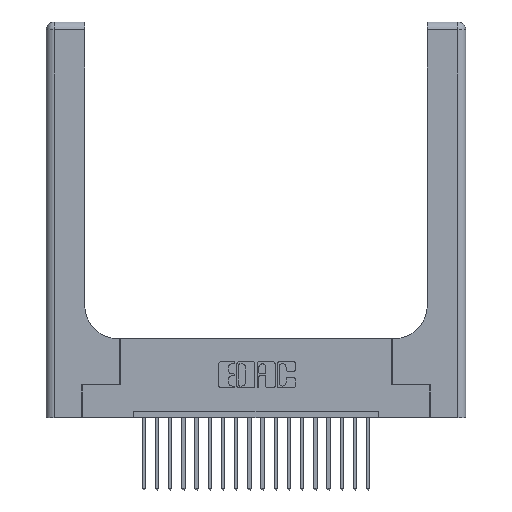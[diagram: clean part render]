
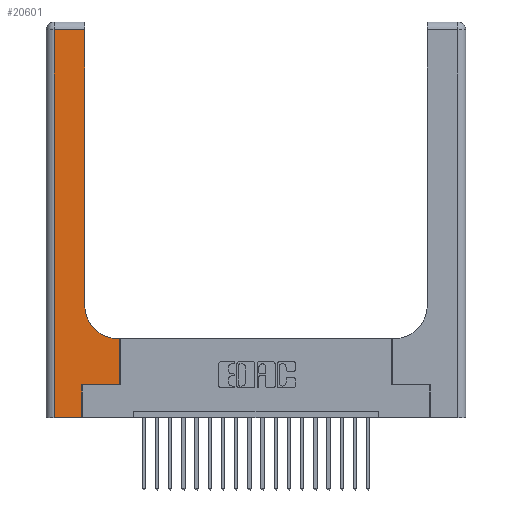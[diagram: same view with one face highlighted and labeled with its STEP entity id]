
A CAD part, top view. The second image highlights one B-rep face of the part: STEP entity #20601.
In plain terms, the highlighted planar face has unit normal (0, 0, 1).
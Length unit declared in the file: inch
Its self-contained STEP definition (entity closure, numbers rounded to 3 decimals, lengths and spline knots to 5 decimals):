
#178 = LINE ( 'NONE', #3616, #10023 ) ;
#368 = EDGE_CURVE ( 'NONE', #13290, #6331, #4164, .T. ) ;
#420 = CARTESIAN_POINT ( 'NONE',  ( 0.06, 3., 0.37 ) ) ;
#850 = AXIS2_PLACEMENT_3D ( 'NONE', #21182, #11050, #14389 ) ;
#1238 = VECTOR ( 'NONE', #5958, 39.37008 ) ;
#1282 = EDGE_CURVE ( 'NONE', #18139, #15798, #9683, .T. ) ;
#2224 = ORIENTED_EDGE ( 'NONE', *, *, #4259, .T. ) ;
#2314 = VECTOR ( 'NONE', #4105, 39.37008 ) ;
#2842 = VERTEX_POINT ( 'NONE', #9582 ) ;
#3616 = CARTESIAN_POINT ( 'NONE',  ( 0.269, 0., 0.37 ) ) ;
#3642 = CARTESIAN_POINT ( 'NONE',  ( 0.06, 0., 0.37 ) ) ;
#3695 = CARTESIAN_POINT ( 'NONE',  ( 0.2915, 3., 0.37 ) ) ;
#3756 = EDGE_LOOP ( 'NONE', ( #5362, #13397, #7333, #3832, #2224, #4231, #17877, #12104, #7374 ) ) ;
#3794 = VECTOR ( 'NONE', #12310, 39.37008 ) ;
#3820 = DIRECTION ( 'NONE',  ( -1., 0., 0. ) ) ;
#3832 = ORIENTED_EDGE ( 'NONE', *, *, #6887, .T. ) ;
#4105 = DIRECTION ( 'NONE',  ( 0., 1., 0. ) ) ;
#4164 = LINE ( 'NONE', #3695, #2314 ) ;
#4189 = EDGE_CURVE ( 'NONE', #15798, #5351, #21672, .T. ) ;
#4231 = ORIENTED_EDGE ( 'NONE', *, *, #1282, .T. ) ;
#4244 = VERTEX_POINT ( 'NONE', #17295 ) ;
#4259 = EDGE_CURVE ( 'NONE', #2842, #18139, #178, .T. ) ;
#4546 = CARTESIAN_POINT ( 'NONE',  ( 0.5585, 0.25, 0.37 ) ) ;
#5351 = VERTEX_POINT ( 'NONE', #12432 ) ;
#5362 = ORIENTED_EDGE ( 'NONE', *, *, #368, .T. ) ;
#5958 = DIRECTION ( 'NONE',  ( 1., 0., 0. ) ) ;
#6331 = VERTEX_POINT ( 'NONE', #7026 ) ;
#6453 = CARTESIAN_POINT ( 'NONE',  ( 0.2915, 0.85, 0.37 ) ) ;
#6887 = EDGE_CURVE ( 'NONE', #18558, #2842, #7539, .T. ) ;
#7026 = CARTESIAN_POINT ( 'NONE',  ( 0.2915, 2.94, 0.37 ) ) ;
#7333 = ORIENTED_EDGE ( 'NONE', *, *, #8013, .T. ) ;
#7374 = ORIENTED_EDGE ( 'NONE', *, *, #14523, .T. ) ;
#7539 = LINE ( 'NONE', #15017, #21849 ) ;
#7588 = CARTESIAN_POINT ( 'NONE',  ( 0.269, 0.25, 0.37 ) ) ;
#7778 = PLANE ( 'NONE',  #850 ) ;
#8013 = EDGE_CURVE ( 'NONE', #4244, #18558, #8259, .T. ) ;
#8259 = LINE ( 'NONE', #420, #3794 ) ;
#8354 = DIRECTION ( 'NONE',  ( 1., 0., 0. ) ) ;
#8928 = DIRECTION ( 'NONE',  ( 0., 1., 0. ) ) ;
#9396 = LINE ( 'NONE', #12491, #17884 ) ;
#9582 = CARTESIAN_POINT ( 'NONE',  ( 0.269, 0., 0.37 ) ) ;
#9683 = LINE ( 'NONE', #7588, #1238 ) ;
#10023 = VECTOR ( 'NONE', #8928, 39.37008 ) ;
#10596 = CARTESIAN_POINT ( 'NONE',  ( 0.5415, 0.6, 0.37 ) ) ;
#10905 = EDGE_CURVE ( 'NONE', #5351, #16462, #15665, .T. ) ;
#11050 = DIRECTION ( 'NONE',  ( 0., 0., -1. ) ) ;
#11297 = CARTESIAN_POINT ( 'NONE',  ( 0.2915, 0.6, 0.37 ) ) ;
#12104 = ORIENTED_EDGE ( 'NONE', *, *, #10905, .T. ) ;
#12310 = DIRECTION ( 'NONE',  ( 0., -1., 0. ) ) ;
#12432 = CARTESIAN_POINT ( 'NONE',  ( 0.5585, 0.6, 0.37 ) ) ;
#12491 = CARTESIAN_POINT ( 'NONE',  ( 0., 2.94, 0.37 ) ) ;
#12860 = AXIS2_PLACEMENT_3D ( 'NONE', #18492, #14949, #8354 ) ;
#12999 = DIRECTION ( 'NONE',  ( -1., 0., 0. ) ) ;
#13147 = CIRCLE ( 'NONE', #12860, 0.25 ) ;
#13290 = VERTEX_POINT ( 'NONE', #6453 ) ;
#13397 = ORIENTED_EDGE ( 'NONE', *, *, #19448, .T. ) ;
#14389 = DIRECTION ( 'NONE',  ( -1., 0., 0. ) ) ;
#14523 = EDGE_CURVE ( 'NONE', #16462, #13290, #13147, .T. ) ;
#14949 = DIRECTION ( 'NONE',  ( 0., 0., -1. ) ) ;
#15017 = CARTESIAN_POINT ( 'NONE',  ( 0., 0., 0.37 ) ) ;
#15660 = DIRECTION ( 'NONE',  ( 0., 1., 0. ) ) ;
#15665 = LINE ( 'NONE', #11297, #20164 ) ;
#15798 = VERTEX_POINT ( 'NONE', #4546 ) ;
#16462 = VERTEX_POINT ( 'NONE', #10596 ) ;
#16905 = VECTOR ( 'NONE', #15660, 39.37008 ) ;
#17295 = CARTESIAN_POINT ( 'NONE',  ( 0.06, 2.94, 0.37 ) ) ;
#17864 = FACE_OUTER_BOUND ( 'NONE', #3756, .T. ) ;
#17877 = ORIENTED_EDGE ( 'NONE', *, *, #4189, .T. ) ;
#17884 = VECTOR ( 'NONE', #3820, 39.37008 ) ;
#18139 = VERTEX_POINT ( 'NONE', #18432 ) ;
#18432 = CARTESIAN_POINT ( 'NONE',  ( 0.269, 0.25, 0.37 ) ) ;
#18492 = CARTESIAN_POINT ( 'NONE',  ( 0.5415, 0.85, 0.37 ) ) ;
#18558 = VERTEX_POINT ( 'NONE', #3642 ) ;
#18911 = CARTESIAN_POINT ( 'NONE',  ( 0.5585, 0.25, 0.37 ) ) ;
#19448 = EDGE_CURVE ( 'NONE', #6331, #4244, #9396, .T. ) ;
#20057 = DIRECTION ( 'NONE',  ( 1., 0., 0. ) ) ;
#20164 = VECTOR ( 'NONE', #12999, 39.37008 ) ;
#20601 = ADVANCED_FACE ( 'NONE', ( #17864 ), #7778, .F. ) ;
#21182 = CARTESIAN_POINT ( 'NONE',  ( 0., 3., 0.37 ) ) ;
#21672 = LINE ( 'NONE', #18911, #16905 ) ;
#21849 = VECTOR ( 'NONE', #20057, 39.37008 ) ;
